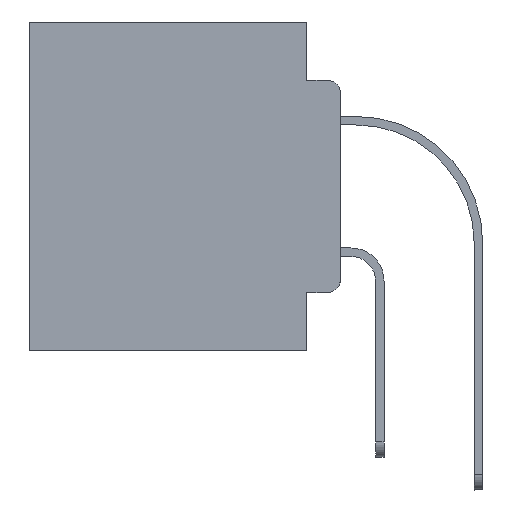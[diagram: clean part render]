
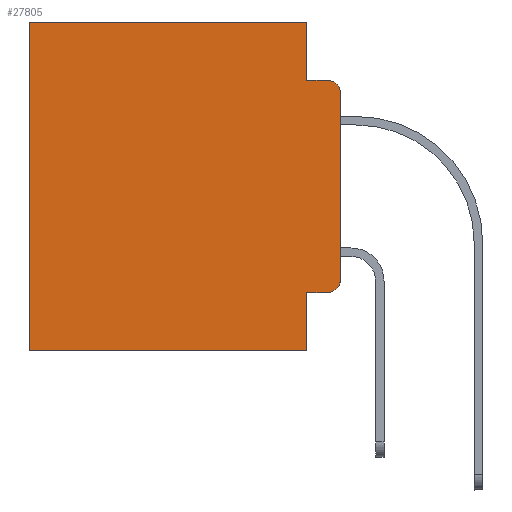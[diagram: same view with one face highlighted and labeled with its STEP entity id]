
A CAD part, left-side view. The second image highlights one B-rep face of the part: STEP entity #27805.
In plain terms, the highlighted planar face has unit normal (-1, 0, 0).
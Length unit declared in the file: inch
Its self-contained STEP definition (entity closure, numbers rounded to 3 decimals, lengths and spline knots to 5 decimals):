
#16 = VERTEX_POINT ( 'NONE', #6740 ) ;
#272 = LINE ( 'NONE', #9336, #15915 ) ;
#1012 = CARTESIAN_POINT ( 'NONE',  ( 0.298, 0., 0. ) ) ;
#1224 = VECTOR ( 'NONE', #18921, 39.37008 ) ;
#1451 = CARTESIAN_POINT ( 'NONE',  ( 0.298, 0.473, 0. ) ) ;
#1702 = ORIENTED_EDGE ( 'NONE', *, *, #20817, .F. ) ;
#2741 = AXIS2_PLACEMENT_3D ( 'NONE', #1012, #10647, #25940 ) ;
#2805 = CARTESIAN_POINT ( 'NONE',  ( 0.298, 0.051, -0.5 ) ) ;
#2866 = ORIENTED_EDGE ( 'NONE', *, *, #13568, .T. ) ;
#2922 = VERTEX_POINT ( 'NONE', #8944 ) ;
#3262 = LINE ( 'NONE', #3851, #26134 ) ;
#3851 = CARTESIAN_POINT ( 'NONE',  ( 0.298, 0.051, -0.4115 ) ) ;
#3925 = AXIS2_PLACEMENT_3D ( 'NONE', #26674, #13148, #22216 ) ;
#4046 = VERTEX_POINT ( 'NONE', #17545 ) ;
#4055 = EDGE_LOOP ( 'NONE', ( #21549, #2866, #1702, #19319, #16443, #12067, #7555, #14667, #7554, #8724 ) ) ;
#4112 = LINE ( 'NONE', #1451, #9279 ) ;
#4702 = CIRCLE ( 'NONE', #21755, 0.02 ) ;
#5295 = DIRECTION ( 'NONE',  ( 0., 0., -1. ) ) ;
#6034 = VERTEX_POINT ( 'NONE', #2805 ) ;
#6054 = EDGE_CURVE ( 'NONE', #27931, #16, #23872, .T. ) ;
#6238 = CARTESIAN_POINT ( 'NONE',  ( 0.298, 0.051, -0.4115 ) ) ;
#6423 = EDGE_CURVE ( 'NONE', #6034, #10566, #8862, .T. ) ;
#6740 = CARTESIAN_POINT ( 'NONE',  ( 0.298, 0.051, -0.0885 ) ) ;
#7057 = VERTEX_POINT ( 'NONE', #6238 ) ;
#7554 = ORIENTED_EDGE ( 'NONE', *, *, #26043, .T. ) ;
#7555 = ORIENTED_EDGE ( 'NONE', *, *, #6423, .F. ) ;
#8374 = DIRECTION ( 'NONE',  ( -1., 0., 0. ) ) ;
#8724 = ORIENTED_EDGE ( 'NONE', *, *, #21147, .T. ) ;
#8862 = LINE ( 'NONE', #22818, #19336 ) ;
#8944 = CARTESIAN_POINT ( 'NONE',  ( 0.298, 0., -0.1085 ) ) ;
#9279 = VECTOR ( 'NONE', #19560, 39.37008 ) ;
#9336 = CARTESIAN_POINT ( 'NONE',  ( 0.298, 0., 0. ) ) ;
#9862 = LINE ( 'NONE', #25597, #1224 ) ;
#10566 = VERTEX_POINT ( 'NONE', #27897 ) ;
#10647 = DIRECTION ( 'NONE',  ( 1., 0., 0. ) ) ;
#10998 = EDGE_CURVE ( 'NONE', #7057, #6034, #25195, .T. ) ;
#12067 = ORIENTED_EDGE ( 'NONE', *, *, #16436, .T. ) ;
#12735 = DIRECTION ( 'NONE',  ( 0., 1., 0. ) ) ;
#13148 = DIRECTION ( 'NONE',  ( -1., 0., 0. ) ) ;
#13394 = VECTOR ( 'NONE', #19701, 39.37008 ) ;
#13454 = DIRECTION ( 'NONE',  ( 0., 1., 0. ) ) ;
#13568 = EDGE_CURVE ( 'NONE', #2922, #17824, #4702, .T. ) ;
#14667 = ORIENTED_EDGE ( 'NONE', *, *, #10998, .F. ) ;
#14997 = CARTESIAN_POINT ( 'NONE',  ( 0.298, 0.02, -0.0885 ) ) ;
#15773 = CIRCLE ( 'NONE', #3925, 0.02 ) ;
#15915 = VECTOR ( 'NONE', #12735, 39.37008 ) ;
#16021 = EDGE_CURVE ( 'NONE', #27931, #4046, #272, .T. ) ;
#16436 = EDGE_CURVE ( 'NONE', #4046, #10566, #4112, .T. ) ;
#16443 = ORIENTED_EDGE ( 'NONE', *, *, #16021, .T. ) ;
#16996 = CARTESIAN_POINT ( 'NONE',  ( 0.298, 0.02, -0.1085 ) ) ;
#17427 = DIRECTION ( 'NONE',  ( 0., 0., -1. ) ) ;
#17467 = FACE_OUTER_BOUND ( 'NONE', #4055, .T. ) ;
#17545 = CARTESIAN_POINT ( 'NONE',  ( 0.298, 0.473, 0. ) ) ;
#17824 = VERTEX_POINT ( 'NONE', #14997 ) ;
#18216 = CARTESIAN_POINT ( 'NONE',  ( 0.298, 0., -0.3915 ) ) ;
#18608 = EDGE_CURVE ( 'NONE', #2922, #19895, #9862, .T. ) ;
#18921 = DIRECTION ( 'NONE',  ( 0., 0., -1. ) ) ;
#19319 = ORIENTED_EDGE ( 'NONE', *, *, #6054, .F. ) ;
#19336 = VECTOR ( 'NONE', #13454, 39.37008 ) ;
#19560 = DIRECTION ( 'NONE',  ( 0., 0., -1. ) ) ;
#19701 = DIRECTION ( 'NONE',  ( 0., -1., 0. ) ) ;
#19895 = VERTEX_POINT ( 'NONE', #18216 ) ;
#20817 = EDGE_CURVE ( 'NONE', #16, #17824, #21925, .T. ) ;
#21147 = EDGE_CURVE ( 'NONE', #23238, #19895, #15773, .T. ) ;
#21549 = ORIENTED_EDGE ( 'NONE', *, *, #18608, .F. ) ;
#21755 = AXIS2_PLACEMENT_3D ( 'NONE', #16996, #8374, #17427 ) ;
#21775 = PLANE ( 'NONE',  #2741 ) ;
#21925 = LINE ( 'NONE', #26381, #13394 ) ;
#22216 = DIRECTION ( 'NONE',  ( 0., 0., -1. ) ) ;
#22652 = CARTESIAN_POINT ( 'NONE',  ( 0.298, 0.051, 0. ) ) ;
#22818 = CARTESIAN_POINT ( 'NONE',  ( 0.298, 0., -0.5 ) ) ;
#22964 = VECTOR ( 'NONE', #5295, 39.37008 ) ;
#23187 = VECTOR ( 'NONE', #28182, 39.37008 ) ;
#23238 = VERTEX_POINT ( 'NONE', #26034 ) ;
#23872 = LINE ( 'NONE', #25516, #23187 ) ;
#25195 = LINE ( 'NONE', #27714, #22964 ) ;
#25516 = CARTESIAN_POINT ( 'NONE',  ( 0.298, 0.051, 0. ) ) ;
#25597 = CARTESIAN_POINT ( 'NONE',  ( 0.298, 0., 0. ) ) ;
#25940 = DIRECTION ( 'NONE',  ( 0., 0., -1. ) ) ;
#26034 = CARTESIAN_POINT ( 'NONE',  ( 0.298, 0.02, -0.4115 ) ) ;
#26043 = EDGE_CURVE ( 'NONE', #7057, #23238, #3262, .T. ) ;
#26134 = VECTOR ( 'NONE', #26559, 39.37008 ) ;
#26381 = CARTESIAN_POINT ( 'NONE',  ( 0.298, 0.051, -0.0885 ) ) ;
#26559 = DIRECTION ( 'NONE',  ( 0., -1., 0. ) ) ;
#26674 = CARTESIAN_POINT ( 'NONE',  ( 0.298, 0.02, -0.3915 ) ) ;
#27714 = CARTESIAN_POINT ( 'NONE',  ( 0.298, 0.051, 0. ) ) ;
#27805 = ADVANCED_FACE ( 'NONE', ( #17467 ), #21775, .F. ) ;
#27897 = CARTESIAN_POINT ( 'NONE',  ( 0.298, 0.473, -0.5 ) ) ;
#27931 = VERTEX_POINT ( 'NONE', #22652 ) ;
#28182 = DIRECTION ( 'NONE',  ( 0., 0., -1. ) ) ;
